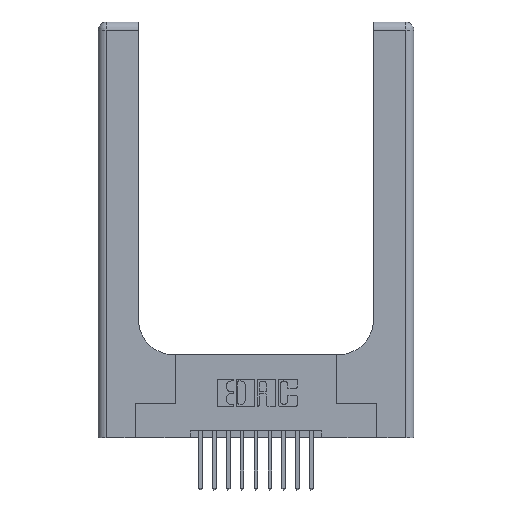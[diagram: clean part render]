
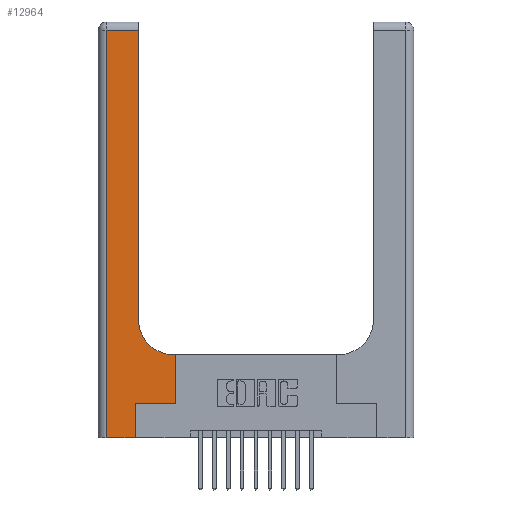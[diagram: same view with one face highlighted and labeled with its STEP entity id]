
A CAD part, top view. The second image highlights one B-rep face of the part: STEP entity #12964.
In plain terms, the highlighted planar face has unit normal (0, 0, 1).
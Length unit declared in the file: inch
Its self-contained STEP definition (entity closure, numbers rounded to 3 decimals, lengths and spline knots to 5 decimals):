
#1409 = VERTEX_POINT ( 'NONE', #15898 ) ;
#1870 = VERTEX_POINT ( 'NONE', #14738 ) ;
#1938 = CARTESIAN_POINT ( 'NONE',  ( 0., 0., 0.37 ) ) ;
#2060 = VERTEX_POINT ( 'NONE', #12512 ) ;
#2152 = CARTESIAN_POINT ( 'NONE',  ( 0.06, 2.94, 0.37 ) ) ;
#2153 = VECTOR ( 'NONE', #13928, 39.37008 ) ;
#2331 = EDGE_LOOP ( 'NONE', ( #5653, #16390, #14195, #12509, #8499, #3595, #5729, #14104, #13605 ) ) ;
#2929 = LINE ( 'NONE', #4887, #12770 ) ;
#2956 = CARTESIAN_POINT ( 'NONE',  ( 0.5585, 0.6, 0.37 ) ) ;
#3158 = LINE ( 'NONE', #13383, #16048 ) ;
#3193 = DIRECTION ( 'NONE',  ( 0., 0., -1. ) ) ;
#3593 = EDGE_CURVE ( 'NONE', #5194, #1409, #14133, .T. ) ;
#3595 = ORIENTED_EDGE ( 'NONE', *, *, #14993, .T. ) ;
#3941 = LINE ( 'NONE', #13131, #6349 ) ;
#4195 = DIRECTION ( 'NONE',  ( -1., 0., 0. ) ) ;
#4598 = DIRECTION ( 'NONE',  ( 0., 0., -1. ) ) ;
#4887 = CARTESIAN_POINT ( 'NONE',  ( 0., 2.94, 0.37 ) ) ;
#4970 = CARTESIAN_POINT ( 'NONE',  ( 0.5585, 0.25, 0.37 ) ) ;
#5194 = VERTEX_POINT ( 'NONE', #14113 ) ;
#5270 = DIRECTION ( 'NONE',  ( 0., -1., 0. ) ) ;
#5294 = LINE ( 'NONE', #14158, #16532 ) ;
#5653 = ORIENTED_EDGE ( 'NONE', *, *, #3593, .T. ) ;
#5729 = ORIENTED_EDGE ( 'NONE', *, *, #7069, .T. ) ;
#5795 = DIRECTION ( 'NONE',  ( -1., 0., 0. ) ) ;
#6084 = VECTOR ( 'NONE', #12783, 39.37008 ) ;
#6286 = CARTESIAN_POINT ( 'NONE',  ( 0.5415, 0.6, 0.37 ) ) ;
#6349 = VECTOR ( 'NONE', #7923, 39.37008 ) ;
#6477 = VERTEX_POINT ( 'NONE', #6286 ) ;
#7009 = AXIS2_PLACEMENT_3D ( 'NONE', #16167, #4598, #12340 ) ;
#7033 = LINE ( 'NONE', #4970, #2153 ) ;
#7069 = EDGE_CURVE ( 'NONE', #2060, #9677, #7033, .T. ) ;
#7125 = CARTESIAN_POINT ( 'NONE',  ( 0.06, 0., 0.37 ) ) ;
#7215 = PLANE ( 'NONE',  #8854 ) ;
#7690 = EDGE_CURVE ( 'NONE', #9677, #6477, #3158, .T. ) ;
#7923 = DIRECTION ( 'NONE',  ( 0., 1., 0. ) ) ;
#7968 = VERTEX_POINT ( 'NONE', #2152 ) ;
#8325 = CARTESIAN_POINT ( 'NONE',  ( 0.269, 0.25, 0.37 ) ) ;
#8499 = ORIENTED_EDGE ( 'NONE', *, *, #12119, .T. ) ;
#8551 = DIRECTION ( 'NONE',  ( 1., 0., 0. ) ) ;
#8854 = AXIS2_PLACEMENT_3D ( 'NONE', #12308, #3193, #5795 ) ;
#9118 = VERTEX_POINT ( 'NONE', #8325 ) ;
#9159 = FACE_OUTER_BOUND ( 'NONE', #2331, .T. ) ;
#9489 = LINE ( 'NONE', #11181, #6084 ) ;
#9677 = VERTEX_POINT ( 'NONE', #2956 ) ;
#10760 = VERTEX_POINT ( 'NONE', #7125 ) ;
#11181 = CARTESIAN_POINT ( 'NONE',  ( 0.269, 0.25, 0.37 ) ) ;
#11478 = CIRCLE ( 'NONE', #7009, 0.25 ) ;
#11480 = EDGE_CURVE ( 'NONE', #1409, #7968, #2929, .T. ) ;
#12119 = EDGE_CURVE ( 'NONE', #1870, #9118, #3941, .T. ) ;
#12308 = CARTESIAN_POINT ( 'NONE',  ( 0., 3., 0.37 ) ) ;
#12340 = DIRECTION ( 'NONE',  ( 1., 0., 0. ) ) ;
#12509 = ORIENTED_EDGE ( 'NONE', *, *, #13039, .T. ) ;
#12512 = CARTESIAN_POINT ( 'NONE',  ( 0.5585, 0.25, 0.37 ) ) ;
#12770 = VECTOR ( 'NONE', #16351, 39.37008 ) ;
#12783 = DIRECTION ( 'NONE',  ( 1., 0., 0. ) ) ;
#12964 = ADVANCED_FACE ( 'NONE', ( #9159 ), #7215, .F. ) ;
#13039 = EDGE_CURVE ( 'NONE', #10760, #1870, #14332, .T. ) ;
#13131 = CARTESIAN_POINT ( 'NONE',  ( 0.269, 0., 0.37 ) ) ;
#13335 = CARTESIAN_POINT ( 'NONE',  ( 0.2915, 3., 0.37 ) ) ;
#13383 = CARTESIAN_POINT ( 'NONE',  ( 0.2915, 0.6, 0.37 ) ) ;
#13605 = ORIENTED_EDGE ( 'NONE', *, *, #15318, .T. ) ;
#13928 = DIRECTION ( 'NONE',  ( 0., 1., 0. ) ) ;
#14104 = ORIENTED_EDGE ( 'NONE', *, *, #7690, .T. ) ;
#14113 = CARTESIAN_POINT ( 'NONE',  ( 0.2915, 0.85, 0.37 ) ) ;
#14133 = LINE ( 'NONE', #13335, #14544 ) ;
#14158 = CARTESIAN_POINT ( 'NONE',  ( 0.06, 3., 0.37 ) ) ;
#14195 = ORIENTED_EDGE ( 'NONE', *, *, #16528, .T. ) ;
#14332 = LINE ( 'NONE', #1938, #14958 ) ;
#14450 = DIRECTION ( 'NONE',  ( 0., 1., 0. ) ) ;
#14544 = VECTOR ( 'NONE', #14450, 39.37008 ) ;
#14738 = CARTESIAN_POINT ( 'NONE',  ( 0.269, 0., 0.37 ) ) ;
#14958 = VECTOR ( 'NONE', #8551, 39.37008 ) ;
#14993 = EDGE_CURVE ( 'NONE', #9118, #2060, #9489, .T. ) ;
#15318 = EDGE_CURVE ( 'NONE', #6477, #5194, #11478, .T. ) ;
#15898 = CARTESIAN_POINT ( 'NONE',  ( 0.2915, 2.94, 0.37 ) ) ;
#16048 = VECTOR ( 'NONE', #4195, 39.37008 ) ;
#16167 = CARTESIAN_POINT ( 'NONE',  ( 0.5415, 0.85, 0.37 ) ) ;
#16351 = DIRECTION ( 'NONE',  ( -1., 0., 0. ) ) ;
#16390 = ORIENTED_EDGE ( 'NONE', *, *, #11480, .T. ) ;
#16528 = EDGE_CURVE ( 'NONE', #7968, #10760, #5294, .T. ) ;
#16532 = VECTOR ( 'NONE', #5270, 39.37008 ) ;
